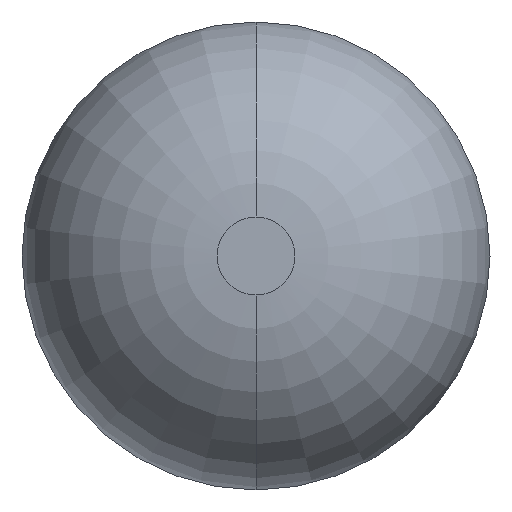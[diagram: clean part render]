
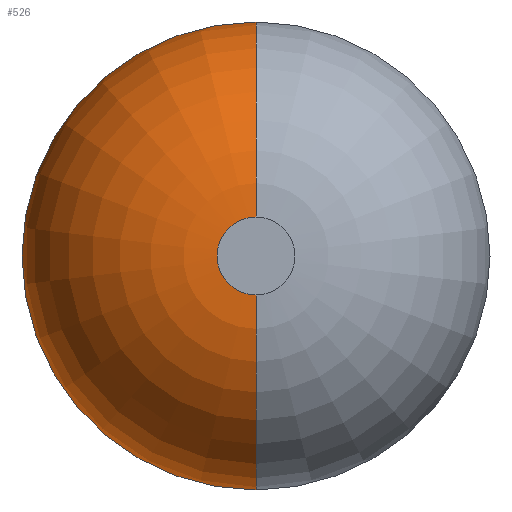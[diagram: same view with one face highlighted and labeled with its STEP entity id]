
A CAD part, left-side view. The second image highlights one B-rep face of the part: STEP entity #526.
In plain terms, the highlighted toroidal (fillet/blend) face has major radius 0.397 mm and minor radius 1.984 mm.
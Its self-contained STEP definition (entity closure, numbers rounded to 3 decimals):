
#45 = DIRECTION ( 'NONE',  ( 0., -1., 0. ) ) ;
#61 = CARTESIAN_POINT ( 'NONE',  ( -10.081, 0., 0. ) ) ;
#72 = VERTEX_POINT ( 'NONE', #394 ) ;
#95 = CIRCLE ( 'NONE', #557, 1.984 ) ;
#97 = CARTESIAN_POINT ( 'NONE',  ( -10.081, 0., 0.397 ) ) ;
#111 = EDGE_CURVE ( 'NONE', #615, #487, #270, .T. ) ;
#112 = CIRCLE ( 'NONE', #649, 2.381 ) ;
#117 = EDGE_CURVE ( 'NONE', #630, #72, #575, .T. ) ;
#125 = CARTESIAN_POINT ( 'NONE',  ( -10.081, 0., 2.381 ) ) ;
#126 = EDGE_CURVE ( 'NONE', #72, #487, #251, .T. ) ;
#129 = EDGE_CURVE ( 'NONE', #212, #615, #112, .T. ) ;
#130 = CARTESIAN_POINT ( 'NONE',  ( -10.081, 0., -0.397 ) ) ;
#136 = CARTESIAN_POINT ( 'NONE',  ( -10.081, 2.381, 0. ) ) ;
#141 = EDGE_CURVE ( 'NONE', #630, #212, #95, .T. ) ;
#150 = CARTESIAN_POINT ( 'NONE',  ( -10.081, 0., 0. ) ) ;
#171 = EDGE_LOOP ( 'NONE', ( #454, #462, #489, #573, #584 ) ) ;
#207 = CARTESIAN_POINT ( 'NONE',  ( -10.081, 0., 0. ) ) ;
#212 = VERTEX_POINT ( 'NONE', #409 ) ;
#213 = DIRECTION ( 'NONE',  ( 0., 1., 0. ) ) ;
#249 = CARTESIAN_POINT ( 'NONE',  ( -12.065, 0., 0. ) ) ;
#251 = CIRCLE ( 'NONE', #652, 1.984 ) ;
#267 = DIRECTION ( 'NONE',  ( 1., 0., 0. ) ) ;
#270 = CIRCLE ( 'NONE', #665, 2.381 ) ;
#283 = DIRECTION ( 'NONE',  ( 0., 0., -1. ) ) ;
#372 = AXIS2_PLACEMENT_3D ( 'NONE', #150, #729, #733 ) ;
#394 = CARTESIAN_POINT ( 'NONE',  ( -12.065, 0., 0.397 ) ) ;
#399 = DIRECTION ( 'NONE',  ( 0., 0., -1. ) ) ;
#409 = CARTESIAN_POINT ( 'NONE',  ( -10.081, 0., -2.381 ) ) ;
#437 = FACE_OUTER_BOUND ( 'NONE', #171, .T. ) ;
#454 = ORIENTED_EDGE ( 'NONE', *, *, #117, .T. ) ;
#462 = ORIENTED_EDGE ( 'NONE', *, *, #126, .T. ) ;
#487 = VERTEX_POINT ( 'NONE', #125 ) ;
#489 = ORIENTED_EDGE ( 'NONE', *, *, #111, .F. ) ;
#507 = DIRECTION ( 'NONE',  ( 0., 0., -1. ) ) ;
#525 = DIRECTION ( 'NONE',  ( 0., 0., -1. ) ) ;
#526 = ADVANCED_FACE ( 'NONE', ( #437 ), #735, .T. ) ;
#553 = DIRECTION ( 'NONE',  ( 1., 0., 0. ) ) ;
#557 = AXIS2_PLACEMENT_3D ( 'NONE', #130, #45, #283 ) ;
#573 = ORIENTED_EDGE ( 'NONE', *, *, #129, .F. ) ;
#575 = CIRCLE ( 'NONE', #658, 0.397 ) ;
#584 = ORIENTED_EDGE ( 'NONE', *, *, #141, .F. ) ;
#615 = VERTEX_POINT ( 'NONE', #136 ) ;
#616 = CARTESIAN_POINT ( 'NONE',  ( -12.065, 0., -0.397 ) ) ;
#630 = VERTEX_POINT ( 'NONE', #616 ) ;
#642 = DIRECTION ( 'NONE',  ( 1., 0., 0. ) ) ;
#649 = AXIS2_PLACEMENT_3D ( 'NONE', #61, #267, #399 ) ;
#652 = AXIS2_PLACEMENT_3D ( 'NONE', #97, #213, #675 ) ;
#658 = AXIS2_PLACEMENT_3D ( 'NONE', #249, #553, #507 ) ;
#665 = AXIS2_PLACEMENT_3D ( 'NONE', #207, #642, #525 ) ;
#675 = DIRECTION ( 'NONE',  ( 0., 0., 1. ) ) ;
#729 = DIRECTION ( 'NONE',  ( 1., 0., 0. ) ) ;
#733 = DIRECTION ( 'NONE',  ( 0., 0., -1. ) ) ;
#735 = TOROIDAL_SURFACE ( 'NONE', #372, 0.397, 1.984 ) ;
